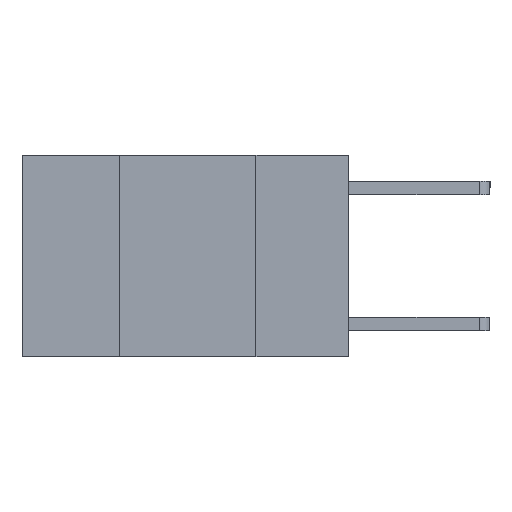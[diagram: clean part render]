
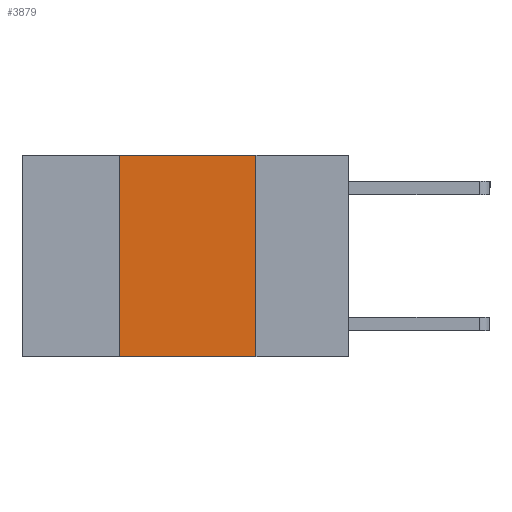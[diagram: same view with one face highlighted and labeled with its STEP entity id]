
A CAD part, left-side view. The second image highlights one B-rep face of the part: STEP entity #3879.
In plain terms, the highlighted planar face has unit normal (-1, 0, 0).
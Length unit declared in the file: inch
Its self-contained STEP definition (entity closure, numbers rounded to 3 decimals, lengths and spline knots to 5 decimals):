
#3 = ORIENTED_EDGE ( 'NONE', *, *, #1207, .F. ) ;
#570 = EDGE_CURVE ( 'NONE', #4890, #4406, #3216, .T. ) ;
#776 = VERTEX_POINT ( 'NONE', #5007 ) ;
#1069 = CARTESIAN_POINT ( 'NONE',  ( 0., 0.42, 0. ) ) ;
#1207 = EDGE_CURVE ( 'NONE', #7728, #4890, #5876, .T. ) ;
#1339 = DIRECTION ( 'NONE',  ( 1., 0., 0. ) ) ;
#1521 = AXIS2_PLACEMENT_3D ( 'NONE', #5041, #1339, #7280 ) ;
#1525 = CARTESIAN_POINT ( 'NONE',  ( 0., 0.42, 0. ) ) ;
#1937 = ORIENTED_EDGE ( 'NONE', *, *, #570, .F. ) ;
#1991 = FACE_OUTER_BOUND ( 'NONE', #2853, .T. ) ;
#2556 = DIRECTION ( 'NONE',  ( 0., -1., 0. ) ) ;
#2814 = VECTOR ( 'NONE', #2556, 39.37008 ) ;
#2853 = EDGE_LOOP ( 'NONE', ( #1937, #3, #5286, #7593 ) ) ;
#3216 = LINE ( 'NONE', #3869, #5649 ) ;
#3580 = VECTOR ( 'NONE', #5723, 39.37008 ) ;
#3869 = CARTESIAN_POINT ( 'NONE',  ( 0., 0.17, 0. ) ) ;
#3879 = ADVANCED_FACE ( 'NONE', ( #1991 ), #4444, .F. ) ;
#4007 = CARTESIAN_POINT ( 'NONE',  ( 0., 0.17, 0. ) ) ;
#4329 = EDGE_CURVE ( 'NONE', #776, #4406, #6656, .T. ) ;
#4406 = VERTEX_POINT ( 'NONE', #6513 ) ;
#4444 = PLANE ( 'NONE',  #1521 ) ;
#4569 = EDGE_CURVE ( 'NONE', #776, #7728, #6215, .T. ) ;
#4890 = VERTEX_POINT ( 'NONE', #4007 ) ;
#5007 = CARTESIAN_POINT ( 'NONE',  ( 0., 0.42, -0.37 ) ) ;
#5041 = CARTESIAN_POINT ( 'NONE',  ( 0., 0.6, 0. ) ) ;
#5286 = ORIENTED_EDGE ( 'NONE', *, *, #4569, .F. ) ;
#5612 = DIRECTION ( 'NONE',  ( 0., 0., 1. ) ) ;
#5649 = VECTOR ( 'NONE', #6904, 39.37008 ) ;
#5654 = VECTOR ( 'NONE', #5612, 39.37008 ) ;
#5723 = DIRECTION ( 'NONE',  ( 0., -1., 0. ) ) ;
#5876 = LINE ( 'NONE', #7326, #2814 ) ;
#5912 = CARTESIAN_POINT ( 'NONE',  ( 0., 0.6, -0.37 ) ) ;
#6215 = LINE ( 'NONE', #1069, #5654 ) ;
#6513 = CARTESIAN_POINT ( 'NONE',  ( 0., 0.17, -0.37 ) ) ;
#6656 = LINE ( 'NONE', #5912, #3580 ) ;
#6904 = DIRECTION ( 'NONE',  ( 0., 0., -1. ) ) ;
#7280 = DIRECTION ( 'NONE',  ( 0., 0., -1. ) ) ;
#7326 = CARTESIAN_POINT ( 'NONE',  ( 0., 0.6, 0. ) ) ;
#7593 = ORIENTED_EDGE ( 'NONE', *, *, #4329, .T. ) ;
#7728 = VERTEX_POINT ( 'NONE', #1525 ) ;
